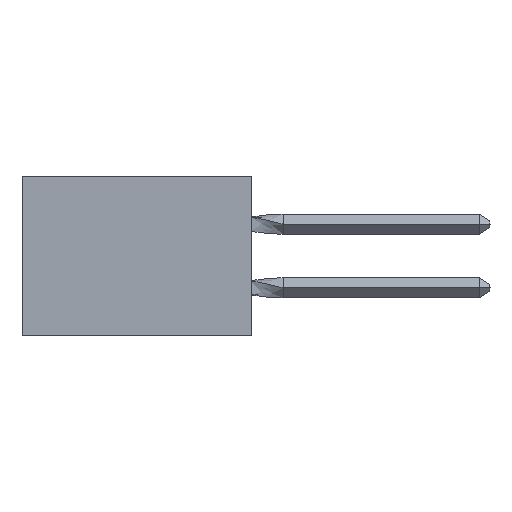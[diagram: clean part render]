
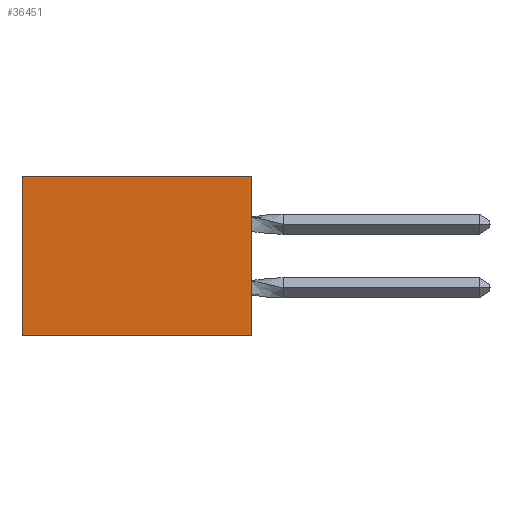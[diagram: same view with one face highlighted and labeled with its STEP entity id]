
A CAD part, left-side view. The second image highlights one B-rep face of the part: STEP entity #36451.
In plain terms, the highlighted planar face has unit normal (-1, 0, 0).
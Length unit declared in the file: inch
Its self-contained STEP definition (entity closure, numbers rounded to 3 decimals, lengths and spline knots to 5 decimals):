
#31 = DIRECTION ( 'NONE',  ( 1., 0., 0. ) ) ;
#159 = VECTOR ( 'NONE', #31886, 39.37008 ) ;
#646 = CARTESIAN_POINT ( 'NONE',  ( 0.305, 0.72, -0.5 ) ) ;
#2605 = CARTESIAN_POINT ( 'NONE',  ( 0.305, 0.72, 0. ) ) ;
#2620 = DIRECTION ( 'NONE',  ( 0., 1., 0. ) ) ;
#3819 = LINE ( 'NONE', #18219, #9823 ) ;
#4537 = ORIENTED_EDGE ( 'NONE', *, *, #18997, .F. ) ;
#5642 = CARTESIAN_POINT ( 'NONE',  ( 0.305, 0., 0. ) ) ;
#6579 = CARTESIAN_POINT ( 'NONE',  ( 0.305, 0., -0.5 ) ) ;
#6792 = ORIENTED_EDGE ( 'NONE', *, *, #25354, .T. ) ;
#8399 = ORIENTED_EDGE ( 'NONE', *, *, #39042, .T. ) ;
#9823 = VECTOR ( 'NONE', #35194, 39.37008 ) ;
#10372 = DIRECTION ( 'NONE',  ( 0., 0., -1. ) ) ;
#12388 = VERTEX_POINT ( 'NONE', #5642 ) ;
#17405 = LINE ( 'NONE', #23379, #40741 ) ;
#17428 = EDGE_LOOP ( 'NONE', ( #6792, #17576, #4537, #8399 ) ) ;
#17576 = ORIENTED_EDGE ( 'NONE', *, *, #33568, .F. ) ;
#18067 = LINE ( 'NONE', #34043, #159 ) ;
#18219 = CARTESIAN_POINT ( 'NONE',  ( 0.305, 0.72, -0.5 ) ) ;
#18997 = EDGE_CURVE ( 'NONE', #12388, #23442, #18067, .T. ) ;
#19933 = VERTEX_POINT ( 'NONE', #646 ) ;
#23379 = CARTESIAN_POINT ( 'NONE',  ( 0.305, 0., -0.5 ) ) ;
#23442 = VERTEX_POINT ( 'NONE', #41274 ) ;
#23766 = VECTOR ( 'NONE', #24719, 39.37008 ) ;
#24719 = DIRECTION ( 'NONE',  ( 0., 1., 0. ) ) ;
#25179 = VERTEX_POINT ( 'NONE', #2605 ) ;
#25354 = EDGE_CURVE ( 'NONE', #25179, #19933, #3819, .T. ) ;
#27910 = CARTESIAN_POINT ( 'NONE',  ( 0.305, 0., 0. ) ) ;
#27986 = FACE_OUTER_BOUND ( 'NONE', #17428, .T. ) ;
#31305 = PLANE ( 'NONE',  #39544 ) ;
#31886 = DIRECTION ( 'NONE',  ( 0., 0., -1. ) ) ;
#33568 = EDGE_CURVE ( 'NONE', #23442, #19933, #17405, .T. ) ;
#34043 = CARTESIAN_POINT ( 'NONE',  ( 0.305, 0., -0.5 ) ) ;
#35194 = DIRECTION ( 'NONE',  ( 0., 0., -1. ) ) ;
#36451 = ADVANCED_FACE ( 'NONE', ( #27986 ), #31305, .F. ) ;
#38984 = LINE ( 'NONE', #27910, #23766 ) ;
#39042 = EDGE_CURVE ( 'NONE', #12388, #25179, #38984, .T. ) ;
#39544 = AXIS2_PLACEMENT_3D ( 'NONE', #6579, #31, #10372 ) ;
#40741 = VECTOR ( 'NONE', #2620, 39.37008 ) ;
#41274 = CARTESIAN_POINT ( 'NONE',  ( 0.305, 0., -0.5 ) ) ;
